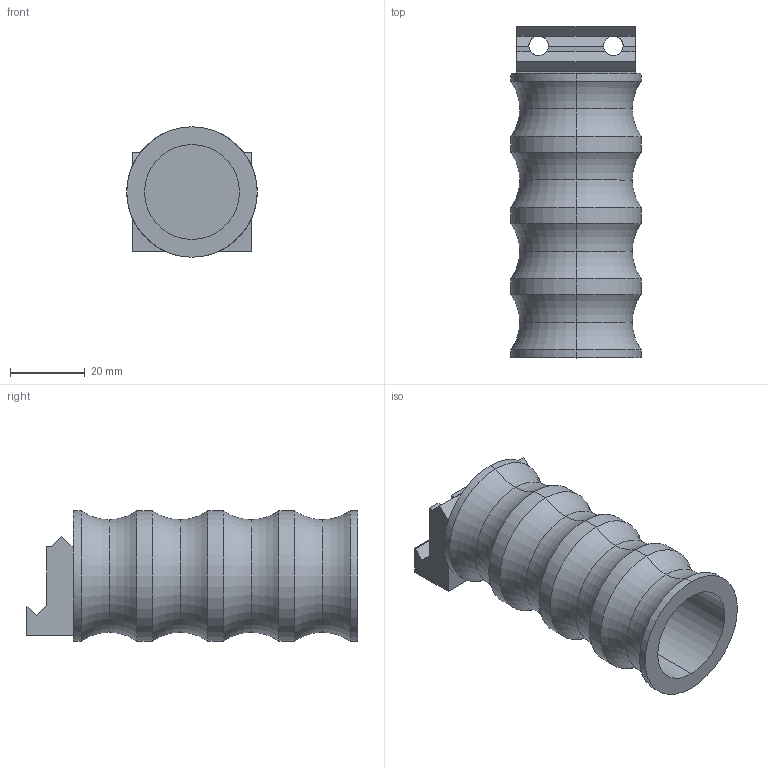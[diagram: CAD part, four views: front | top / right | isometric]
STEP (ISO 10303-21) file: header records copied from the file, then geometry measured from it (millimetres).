
FILE_DESCRIPTION (( 'STEP AP203' ), '1' );
FILE_NAME ('ForeGrip.STEP', '2012-04-22T16:13:50', ( '' ), ( '' ), 'SwSTEP 2.0', 'SolidWorks 2012', '' );
FILE_SCHEMA (( 'CONFIG_CONTROL_DESIGN' ));
Length unit declared in the file: inch
Products named in the file (1): ForeGrip
Bounding box: 34.92 x 88.9 x 34.92 mm (x, y, z)
Volume: 33846.5 mm3; surface area: 17371.7 mm2
Topology: 1 solids, 1 shells, 60 faces, 145 edges, 86 vertices
Faces by surface type: plane 28, torus 16, cylinder 16
Entity records: 1824 total; most frequent: CARTESIAN_POINT 328, DIRECTION 319, ORIENTED_EDGE 290, EDGE_CURVE 145, AXIS2_PLACEMENT_3D 125, VERTEX_POINT 86, LINE 69, VECTOR 69
